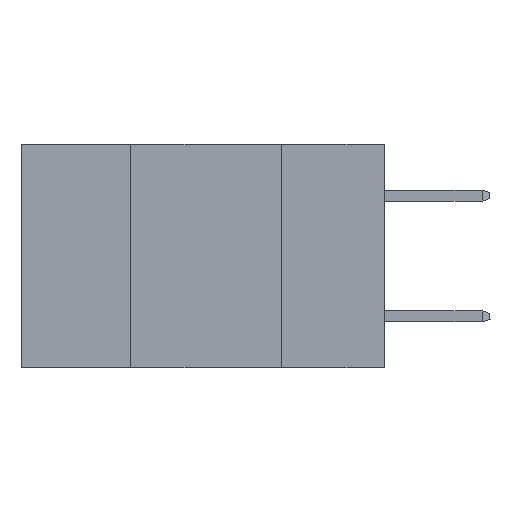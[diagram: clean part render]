
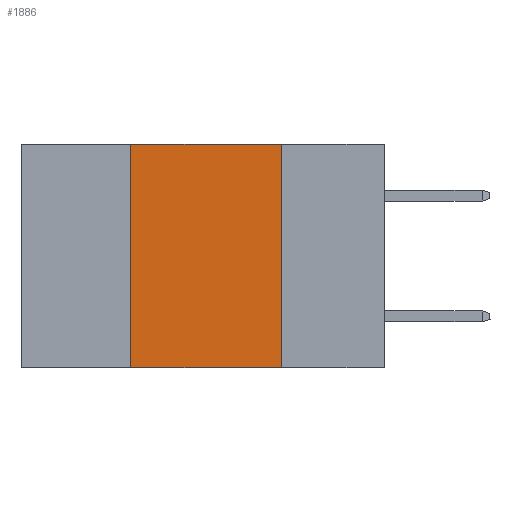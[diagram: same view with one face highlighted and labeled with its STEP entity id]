
A CAD part, left-side view. The second image highlights one B-rep face of the part: STEP entity #1886.
In plain terms, the highlighted planar face has unit normal (-1, 0, 0).
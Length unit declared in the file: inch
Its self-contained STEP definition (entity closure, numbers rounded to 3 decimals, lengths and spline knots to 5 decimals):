
#1088 = CARTESIAN_POINT ( 'NONE',  ( 0., 0.6, 0. ) ) ;
#1146 = LINE ( 'NONE', #13363, #15061 ) ;
#1886 = ADVANCED_FACE ( 'NONE', ( #13532 ), #13397, .F. ) ;
#2125 = LINE ( 'NONE', #10411, #8896 ) ;
#3047 = EDGE_CURVE ( 'NONE', #3774, #7850, #2125, .T. ) ;
#3774 = VERTEX_POINT ( 'NONE', #17154 ) ;
#5136 = AXIS2_PLACEMENT_3D ( 'NONE', #10314, #9209, #8977 ) ;
#5240 = DIRECTION ( 'NONE',  ( 0., -1., 0. ) ) ;
#5546 = VERTEX_POINT ( 'NONE', #13568 ) ;
#6486 = EDGE_CURVE ( 'NONE', #5546, #9398, #1146, .T. ) ;
#7850 = VERTEX_POINT ( 'NONE', #12322 ) ;
#8896 = VECTOR ( 'NONE', #10074, 39.37008 ) ;
#8977 = DIRECTION ( 'NONE',  ( 0., 0., -1. ) ) ;
#9209 = DIRECTION ( 'NONE',  ( 1., 0., 0. ) ) ;
#9398 = VERTEX_POINT ( 'NONE', #16640 ) ;
#10074 = DIRECTION ( 'NONE',  ( 0., 0., 1. ) ) ;
#10314 = CARTESIAN_POINT ( 'NONE',  ( 0., 0.6, 0. ) ) ;
#10411 = CARTESIAN_POINT ( 'NONE',  ( 0., 0.42, -0.37 ) ) ;
#11807 = CARTESIAN_POINT ( 'NONE',  ( 0., 0.6, -0.37 ) ) ;
#12103 = LINE ( 'NONE', #1088, #15269 ) ;
#12164 = EDGE_LOOP ( 'NONE', ( #12294, #14582, #15034, #16672 ) ) ;
#12294 = ORIENTED_EDGE ( 'NONE', *, *, #6486, .F. ) ;
#12322 = CARTESIAN_POINT ( 'NONE',  ( 0., 0.42, 0. ) ) ;
#12585 = EDGE_CURVE ( 'NONE', #7850, #5546, #12103, .T. ) ;
#12680 = VECTOR ( 'NONE', #13171, 39.37008 ) ;
#13171 = DIRECTION ( 'NONE',  ( 0., -1., 0. ) ) ;
#13186 = DIRECTION ( 'NONE',  ( 0., 0., -1. ) ) ;
#13363 = CARTESIAN_POINT ( 'NONE',  ( 0., 0.17, -0.37 ) ) ;
#13397 = PLANE ( 'NONE',  #5136 ) ;
#13532 = FACE_OUTER_BOUND ( 'NONE', #12164, .T. ) ;
#13568 = CARTESIAN_POINT ( 'NONE',  ( 0., 0.17, 0. ) ) ;
#14061 = EDGE_CURVE ( 'NONE', #3774, #9398, #16635, .T. ) ;
#14582 = ORIENTED_EDGE ( 'NONE', *, *, #12585, .F. ) ;
#15034 = ORIENTED_EDGE ( 'NONE', *, *, #3047, .F. ) ;
#15061 = VECTOR ( 'NONE', #13186, 39.37008 ) ;
#15269 = VECTOR ( 'NONE', #5240, 39.37008 ) ;
#16635 = LINE ( 'NONE', #11807, #12680 ) ;
#16640 = CARTESIAN_POINT ( 'NONE',  ( 0., 0.17, -0.37 ) ) ;
#16672 = ORIENTED_EDGE ( 'NONE', *, *, #14061, .T. ) ;
#17154 = CARTESIAN_POINT ( 'NONE',  ( 0., 0.42, -0.37 ) ) ;
